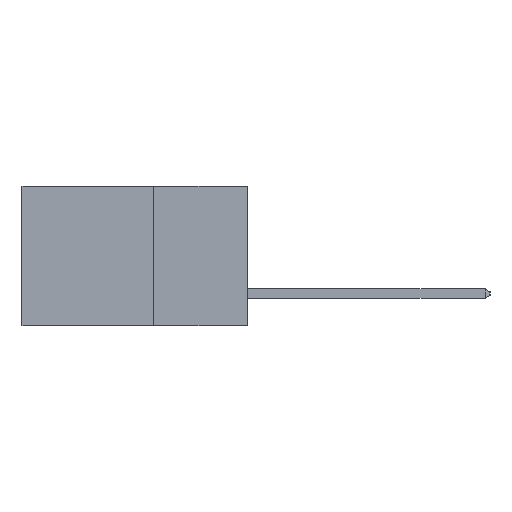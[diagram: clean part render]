
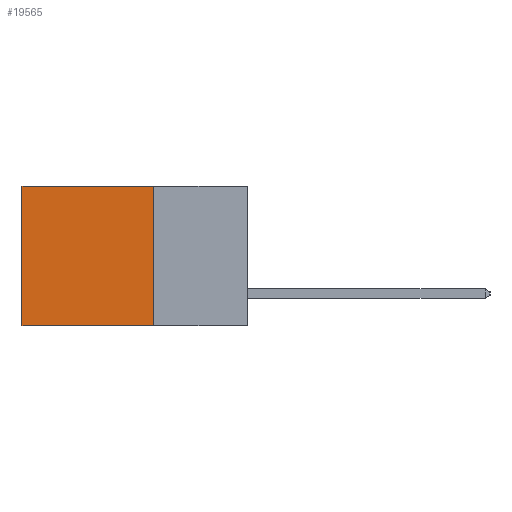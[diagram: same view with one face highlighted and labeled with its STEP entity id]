
A CAD part, left-side view. The second image highlights one B-rep face of the part: STEP entity #19565.
In plain terms, the highlighted planar face has unit normal (-1, 0, 0).
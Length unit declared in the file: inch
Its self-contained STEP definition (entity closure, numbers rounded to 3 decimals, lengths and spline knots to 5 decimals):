
#186 = FACE_OUTER_BOUND ( 'NONE', #1205, .T. ) ;
#865 = CARTESIAN_POINT ( 'NONE',  ( 0.2615, 0.25, -0.37 ) ) ;
#883 = CARTESIAN_POINT ( 'NONE',  ( 0.2615, 0.25, -0.37 ) ) ;
#1205 = EDGE_LOOP ( 'NONE', ( #15650, #3554, #4341, #24552 ) ) ;
#1224 = CARTESIAN_POINT ( 'NONE',  ( 0.2615, 0.6, 0. ) ) ;
#1409 = VECTOR ( 'NONE', #12766, 39.37008 ) ;
#2271 = LINE ( 'NONE', #883, #23025 ) ;
#2446 = CARTESIAN_POINT ( 'NONE',  ( 0.2615, 0.25, 0. ) ) ;
#2844 = EDGE_CURVE ( 'NONE', #17291, #18911, #24079, .T. ) ;
#3405 = EDGE_CURVE ( 'NONE', #7859, #17291, #17290, .T. ) ;
#3554 = ORIENTED_EDGE ( 'NONE', *, *, #22128, .F. ) ;
#4341 = ORIENTED_EDGE ( 'NONE', *, *, #17790, .F. ) ;
#5935 = DIRECTION ( 'NONE',  ( 0., 0., -1. ) ) ;
#6041 = CARTESIAN_POINT ( 'NONE',  ( 0.2615, 0.6, -0.37 ) ) ;
#6434 = PLANE ( 'NONE',  #19654 ) ;
#7859 = VERTEX_POINT ( 'NONE', #2446 ) ;
#8562 = CARTESIAN_POINT ( 'NONE',  ( 0.2615, 0.6, -0.37 ) ) ;
#8716 = VECTOR ( 'NONE', #5935, 39.37008 ) ;
#9288 = DIRECTION ( 'NONE',  ( 0., 1., 0. ) ) ;
#10430 = CARTESIAN_POINT ( 'NONE',  ( 0.2615, 0.25, 0. ) ) ;
#10442 = DIRECTION ( 'NONE',  ( 0., 0., -1. ) ) ;
#10816 = DIRECTION ( 'NONE',  ( 0., 1., 0. ) ) ;
#11957 = LINE ( 'NONE', #865, #1409 ) ;
#12766 = DIRECTION ( 'NONE',  ( 0., 0., -1. ) ) ;
#15650 = ORIENTED_EDGE ( 'NONE', *, *, #2844, .T. ) ;
#15833 = CARTESIAN_POINT ( 'NONE',  ( 0.2615, 0.25, -0.37 ) ) ;
#17290 = LINE ( 'NONE', #10430, #21766 ) ;
#17291 = VERTEX_POINT ( 'NONE', #1224 ) ;
#17790 = EDGE_CURVE ( 'NONE', #7859, #20726, #11957, .T. ) ;
#18911 = VERTEX_POINT ( 'NONE', #8562 ) ;
#19565 = ADVANCED_FACE ( 'NONE', ( #186 ), #6434, .F. ) ;
#19654 = AXIS2_PLACEMENT_3D ( 'NONE', #20162, #22037, #10442 ) ;
#20162 = CARTESIAN_POINT ( 'NONE',  ( 0.2615, 0.25, -0.37 ) ) ;
#20726 = VERTEX_POINT ( 'NONE', #15833 ) ;
#21766 = VECTOR ( 'NONE', #9288, 39.37008 ) ;
#22037 = DIRECTION ( 'NONE',  ( 1., 0., 0. ) ) ;
#22128 = EDGE_CURVE ( 'NONE', #20726, #18911, #2271, .T. ) ;
#23025 = VECTOR ( 'NONE', #10816, 39.37008 ) ;
#24079 = LINE ( 'NONE', #6041, #8716 ) ;
#24552 = ORIENTED_EDGE ( 'NONE', *, *, #3405, .T. ) ;
